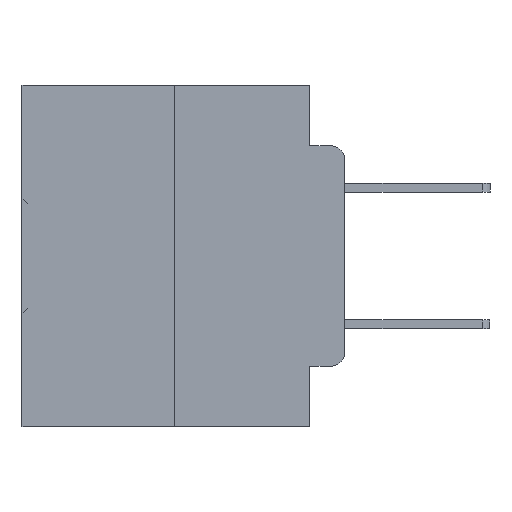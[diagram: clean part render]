
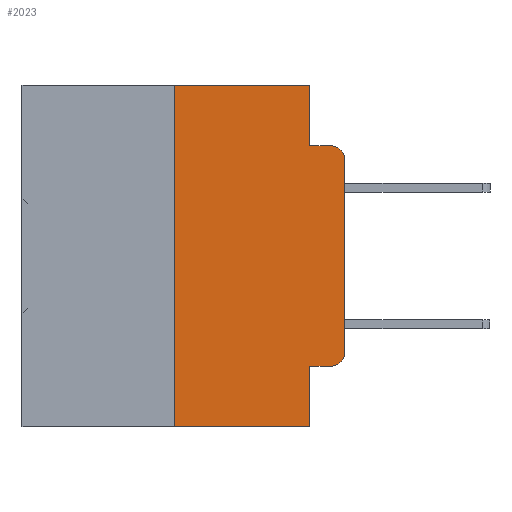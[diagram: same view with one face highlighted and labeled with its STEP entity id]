
A CAD part, left-side view. The second image highlights one B-rep face of the part: STEP entity #2023.
In plain terms, the highlighted planar face has unit normal (-1, 0, 0).
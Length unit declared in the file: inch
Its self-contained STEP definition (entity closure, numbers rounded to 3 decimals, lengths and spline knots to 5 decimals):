
#219 = CIRCLE ( 'NONE', #2981, 0.02 ) ;
#437 = CARTESIAN_POINT ( 'NONE',  ( 0., 0.051, -0.4115 ) ) ;
#478 = ORIENTED_EDGE ( 'NONE', *, *, #32369, .T. ) ;
#952 = CARTESIAN_POINT ( 'NONE',  ( 0., 0.25, 0. ) ) ;
#2023 = ADVANCED_FACE ( 'NONE', ( #25873 ), #2325, .F. ) ;
#2263 = EDGE_CURVE ( 'NONE', #25649, #34565, #3967, .T. ) ;
#2325 = PLANE ( 'NONE',  #24366 ) ;
#2521 = ORIENTED_EDGE ( 'NONE', *, *, #16319, .F. ) ;
#2981 = AXIS2_PLACEMENT_3D ( 'NONE', #19276, #3064, #21951 ) ;
#3064 = DIRECTION ( 'NONE',  ( -1., 0., 0. ) ) ;
#3967 = LINE ( 'NONE', #24585, #10278 ) ;
#4413 = ORIENTED_EDGE ( 'NONE', *, *, #18199, .T. ) ;
#5946 = CARTESIAN_POINT ( 'NONE',  ( 0., 0.473, 0. ) ) ;
#5992 = DIRECTION ( 'NONE',  ( 0., -1., 0. ) ) ;
#6063 = CARTESIAN_POINT ( 'NONE',  ( 0., 0., 0. ) ) ;
#6305 = DIRECTION ( 'NONE',  ( 0., 0., -1. ) ) ;
#6471 = DIRECTION ( 'NONE',  ( 0., 0., 1. ) ) ;
#6707 = EDGE_CURVE ( 'NONE', #17553, #34565, #19357, .T. ) ;
#8090 = ORIENTED_EDGE ( 'NONE', *, *, #6707, .F. ) ;
#8416 = VECTOR ( 'NONE', #8643, 39.37008 ) ;
#8643 = DIRECTION ( 'NONE',  ( 0., -1., 0. ) ) ;
#8758 = DIRECTION ( 'NONE',  ( 0., 0., 1. ) ) ;
#8886 = VERTEX_POINT ( 'NONE', #34051 ) ;
#9424 = CARTESIAN_POINT ( 'NONE',  ( 0., 0.051, -0.0885 ) ) ;
#9471 = CARTESIAN_POINT ( 'NONE',  ( 0., 0.473, 0. ) ) ;
#9700 = DIRECTION ( 'NONE',  ( 1., 0., 0. ) ) ;
#9784 = CIRCLE ( 'NONE', #25075, 0.02 ) ;
#9843 = VERTEX_POINT ( 'NONE', #32756 ) ;
#10278 = VECTOR ( 'NONE', #12586, 39.37008 ) ;
#10492 = CARTESIAN_POINT ( 'NONE',  ( 0., 0.051, -0.0885 ) ) ;
#11548 = VERTEX_POINT ( 'NONE', #10492 ) ;
#12129 = DIRECTION ( 'NONE',  ( 0., -1., 0. ) ) ;
#12338 = CARTESIAN_POINT ( 'NONE',  ( 0., 0.25, -0.5 ) ) ;
#12539 = LINE ( 'NONE', #6063, #25992 ) ;
#12586 = DIRECTION ( 'NONE',  ( 0., -1., 0. ) ) ;
#13196 = EDGE_CURVE ( 'NONE', #25435, #11548, #33168, .T. ) ;
#13689 = EDGE_LOOP ( 'NONE', ( #34175, #28496, #21113, #18160, #26958, #2521, #14067, #8090, #478, #4413 ) ) ;
#14067 = ORIENTED_EDGE ( 'NONE', *, *, #2263, .T. ) ;
#14316 = VECTOR ( 'NONE', #6471, 39.37008 ) ;
#15047 = DIRECTION ( 'NONE',  ( 0., 0., -1. ) ) ;
#15213 = LINE ( 'NONE', #22132, #22378 ) ;
#15750 = CARTESIAN_POINT ( 'NONE',  ( 0., 0.02, -0.1085 ) ) ;
#16001 = VECTOR ( 'NONE', #12129, 39.37008 ) ;
#16133 = DIRECTION ( 'NONE',  ( 0., 0., -1. ) ) ;
#16319 = EDGE_CURVE ( 'NONE', #25649, #9843, #28498, .T. ) ;
#17553 = VERTEX_POINT ( 'NONE', #437 ) ;
#18049 = CARTESIAN_POINT ( 'NONE',  ( 0., 0.02, -0.0885 ) ) ;
#18160 = ORIENTED_EDGE ( 'NONE', *, *, #13196, .F. ) ;
#18199 = EDGE_CURVE ( 'NONE', #30638, #8886, #219, .T. ) ;
#18373 = VECTOR ( 'NONE', #15047, 39.37008 ) ;
#18486 = DIRECTION ( 'NONE',  ( 0., 0., -1. ) ) ;
#19039 = CARTESIAN_POINT ( 'NONE',  ( 0., 0.02, -0.4115 ) ) ;
#19276 = CARTESIAN_POINT ( 'NONE',  ( 0., 0.02, -0.3915 ) ) ;
#19357 = LINE ( 'NONE', #29382, #32516 ) ;
#21113 = ORIENTED_EDGE ( 'NONE', *, *, #33209, .F. ) ;
#21592 = VERTEX_POINT ( 'NONE', #18049 ) ;
#21951 = DIRECTION ( 'NONE',  ( 0., 0., -1. ) ) ;
#22132 = CARTESIAN_POINT ( 'NONE',  ( 0., 0.051, -0.4115 ) ) ;
#22378 = VECTOR ( 'NONE', #5992, 39.37008 ) ;
#22732 = LINE ( 'NONE', #5946, #8416 ) ;
#23047 = CARTESIAN_POINT ( 'NONE',  ( 0., 0., -0.1085 ) ) ;
#24366 = AXIS2_PLACEMENT_3D ( 'NONE', #9471, #9700, #6305 ) ;
#24585 = CARTESIAN_POINT ( 'NONE',  ( 0., 0.473, -0.5 ) ) ;
#24815 = LINE ( 'NONE', #9424, #16001 ) ;
#25075 = AXIS2_PLACEMENT_3D ( 'NONE', #15750, #34203, #18486 ) ;
#25313 = CARTESIAN_POINT ( 'NONE',  ( 0., 0.051, 0. ) ) ;
#25331 = EDGE_CURVE ( 'NONE', #8886, #26316, #12539, .T. ) ;
#25435 = VERTEX_POINT ( 'NONE', #25313 ) ;
#25649 = VERTEX_POINT ( 'NONE', #12338 ) ;
#25813 = CARTESIAN_POINT ( 'NONE',  ( 0., 0.051, 0. ) ) ;
#25873 = FACE_OUTER_BOUND ( 'NONE', #13689, .T. ) ;
#25916 = CARTESIAN_POINT ( 'NONE',  ( 0., 0.051, -0.5 ) ) ;
#25992 = VECTOR ( 'NONE', #8758, 39.37008 ) ;
#26316 = VERTEX_POINT ( 'NONE', #23047 ) ;
#26451 = EDGE_CURVE ( 'NONE', #26316, #21592, #9784, .T. ) ;
#26958 = ORIENTED_EDGE ( 'NONE', *, *, #33003, .F. ) ;
#28496 = ORIENTED_EDGE ( 'NONE', *, *, #26451, .T. ) ;
#28498 = LINE ( 'NONE', #952, #14316 ) ;
#29382 = CARTESIAN_POINT ( 'NONE',  ( 0., 0.051, 0. ) ) ;
#30638 = VERTEX_POINT ( 'NONE', #19039 ) ;
#32369 = EDGE_CURVE ( 'NONE', #17553, #30638, #15213, .T. ) ;
#32516 = VECTOR ( 'NONE', #16133, 39.37008 ) ;
#32756 = CARTESIAN_POINT ( 'NONE',  ( 0., 0.25, 0. ) ) ;
#33003 = EDGE_CURVE ( 'NONE', #9843, #25435, #22732, .T. ) ;
#33168 = LINE ( 'NONE', #25813, #18373 ) ;
#33209 = EDGE_CURVE ( 'NONE', #11548, #21592, #24815, .T. ) ;
#34051 = CARTESIAN_POINT ( 'NONE',  ( 0., 0., -0.3915 ) ) ;
#34175 = ORIENTED_EDGE ( 'NONE', *, *, #25331, .T. ) ;
#34203 = DIRECTION ( 'NONE',  ( -1., 0., 0. ) ) ;
#34565 = VERTEX_POINT ( 'NONE', #25916 ) ;
